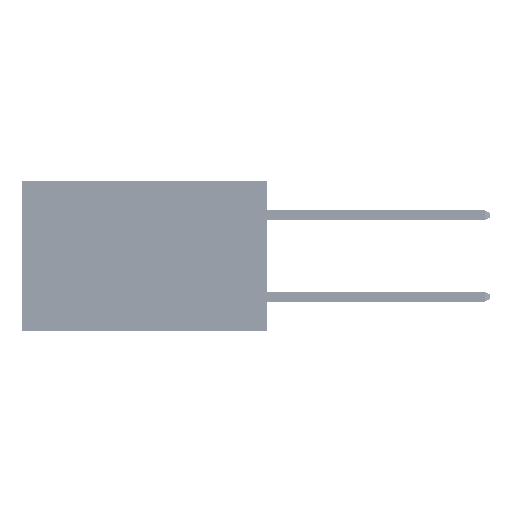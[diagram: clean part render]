
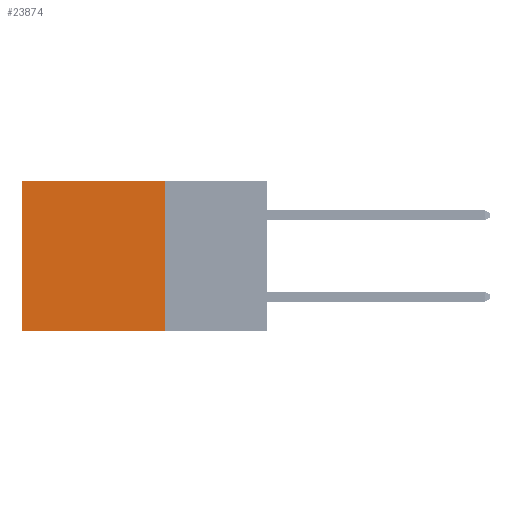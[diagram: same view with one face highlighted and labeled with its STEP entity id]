
A CAD part, left-side view. The second image highlights one B-rep face of the part: STEP entity #23874.
In plain terms, the highlighted planar face has unit normal (-1, 0, 0).
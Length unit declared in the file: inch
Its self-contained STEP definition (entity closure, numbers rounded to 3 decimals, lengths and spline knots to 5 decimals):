
#66 = DIRECTION ( 'NONE',  ( 0., 1., 0. ) ) ;
#891 = EDGE_LOOP ( 'NONE', ( #20433, #35957, #18141, #29507 ) ) ;
#4391 = VERTEX_POINT ( 'NONE', #35763 ) ;
#6802 = PLANE ( 'NONE',  #48245 ) ;
#7699 = CARTESIAN_POINT ( 'NONE',  ( 0.2875, 0.6, 0. ) ) ;
#8863 = VERTEX_POINT ( 'NONE', #26716 ) ;
#8963 = EDGE_CURVE ( 'NONE', #8863, #4391, #16332, .T. ) ;
#14815 = DIRECTION ( 'NONE',  ( 0., 0., -1. ) ) ;
#16332 = LINE ( 'NONE', #31047, #47908 ) ;
#16927 = VERTEX_POINT ( 'NONE', #46619 ) ;
#18061 = EDGE_CURVE ( 'NONE', #4391, #16927, #20159, .T. ) ;
#18141 = ORIENTED_EDGE ( 'NONE', *, *, #32235, .F. ) ;
#18730 = EDGE_CURVE ( 'NONE', #33981, #16927, #39790, .T. ) ;
#18979 = DIRECTION ( 'NONE',  ( 0., 1., 0. ) ) ;
#19469 = VECTOR ( 'NONE', #18979, 39.37008 ) ;
#20159 = LINE ( 'NONE', #7699, #30336 ) ;
#20433 = ORIENTED_EDGE ( 'NONE', *, *, #18061, .T. ) ;
#23874 = ADVANCED_FACE ( 'NONE', ( #28102 ), #6802, .F. ) ;
#26716 = CARTESIAN_POINT ( 'NONE',  ( 0.2875, 0.25, 0. ) ) ;
#28102 = FACE_OUTER_BOUND ( 'NONE', #891, .T. ) ;
#29507 = ORIENTED_EDGE ( 'NONE', *, *, #8963, .T. ) ;
#30336 = VECTOR ( 'NONE', #34757, 39.37008 ) ;
#30529 = CARTESIAN_POINT ( 'NONE',  ( 0.2875, 0.25, -0.37 ) ) ;
#31047 = CARTESIAN_POINT ( 'NONE',  ( 0.2875, 0.25, 0. ) ) ;
#32235 = EDGE_CURVE ( 'NONE', #8863, #33981, #35430, .T. ) ;
#33894 = CARTESIAN_POINT ( 'NONE',  ( 0.2875, 0.25, 0. ) ) ;
#33981 = VERTEX_POINT ( 'NONE', #47227 ) ;
#34757 = DIRECTION ( 'NONE',  ( 0., 0., -1. ) ) ;
#35430 = LINE ( 'NONE', #37783, #44295 ) ;
#35763 = CARTESIAN_POINT ( 'NONE',  ( 0.2875, 0.6, 0. ) ) ;
#35957 = ORIENTED_EDGE ( 'NONE', *, *, #18730, .F. ) ;
#37734 = DIRECTION ( 'NONE',  ( 1., 0., 0. ) ) ;
#37783 = CARTESIAN_POINT ( 'NONE',  ( 0.2875, 0.25, 0. ) ) ;
#39790 = LINE ( 'NONE', #30529, #19469 ) ;
#41575 = DIRECTION ( 'NONE',  ( 0., 0., -1. ) ) ;
#44295 = VECTOR ( 'NONE', #41575, 39.37008 ) ;
#46619 = CARTESIAN_POINT ( 'NONE',  ( 0.2875, 0.6, -0.37 ) ) ;
#47227 = CARTESIAN_POINT ( 'NONE',  ( 0.2875, 0.25, -0.37 ) ) ;
#47908 = VECTOR ( 'NONE', #66, 39.37008 ) ;
#48245 = AXIS2_PLACEMENT_3D ( 'NONE', #33894, #37734, #14815 ) ;
